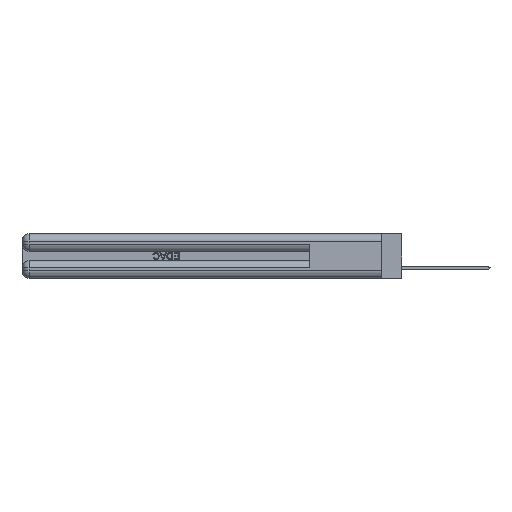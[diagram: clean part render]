
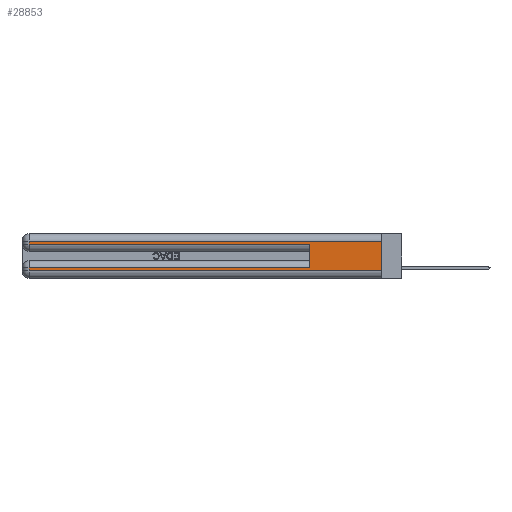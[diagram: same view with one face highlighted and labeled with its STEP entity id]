
A CAD part, left-side view. The second image highlights one B-rep face of the part: STEP entity #28853.
In plain terms, the highlighted planar face has unit normal (-1, 0, 0).
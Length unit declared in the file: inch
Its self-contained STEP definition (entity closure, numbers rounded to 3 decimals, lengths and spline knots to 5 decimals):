
#26 = EDGE_CURVE ( 'NONE', #20165, #24539, #9355, .T. ) ;
#175 = LINE ( 'NONE', #1362, #8796 ) ;
#1362 = CARTESIAN_POINT ( 'NONE',  ( 0., 0., 0.06 ) ) ;
#1652 = CARTESIAN_POINT ( 'NONE',  ( 0., 0.6, 0.145 ) ) ;
#2796 = VECTOR ( 'NONE', #25248, 39.37008 ) ;
#2855 = LINE ( 'NONE', #46911, #2796 ) ;
#3890 = CARTESIAN_POINT ( 'NONE',  ( 0., 2.94, 0.085 ) ) ;
#4137 = PLANE ( 'NONE',  #33162 ) ;
#4166 = CARTESIAN_POINT ( 'NONE',  ( 0., 0., 0.31 ) ) ;
#4442 = EDGE_CURVE ( 'NONE', #18019, #33013, #18798, .T. ) ;
#5843 = VERTEX_POINT ( 'NONE', #46590 ) ;
#6129 = ORIENTED_EDGE ( 'NONE', *, *, #8748, .T. ) ;
#6466 = ORIENTED_EDGE ( 'NONE', *, *, #26, .T. ) ;
#6897 = VECTOR ( 'NONE', #45679, 39.37008 ) ;
#8748 = EDGE_CURVE ( 'NONE', #40566, #5843, #175, .T. ) ;
#8796 = VECTOR ( 'NONE', #26908, 39.37008 ) ;
#9355 = LINE ( 'NONE', #15048, #45819 ) ;
#10079 = VECTOR ( 'NONE', #32707, 39.37008 ) ;
#11359 = EDGE_CURVE ( 'NONE', #24539, #33013, #2855, .T. ) ;
#11821 = CARTESIAN_POINT ( 'NONE',  ( 0., 0.6, 0.285 ) ) ;
#12032 = VERTEX_POINT ( 'NONE', #4166 ) ;
#14096 = EDGE_CURVE ( 'NONE', #45176, #40566, #24363, .T. ) ;
#15048 = CARTESIAN_POINT ( 'NONE',  ( 0., 2.94, 0.37 ) ) ;
#16114 = CARTESIAN_POINT ( 'NONE',  ( 0., 2.94, 0.31 ) ) ;
#16391 = CARTESIAN_POINT ( 'NONE',  ( 0., 2.94, 0.285 ) ) ;
#16403 = CARTESIAN_POINT ( 'NONE',  ( 0., 0., 0.31 ) ) ;
#17459 = LINE ( 'NONE', #28506, #28303 ) ;
#18019 = VERTEX_POINT ( 'NONE', #44288 ) ;
#18798 = LINE ( 'NONE', #1652, #34132 ) ;
#20165 = VERTEX_POINT ( 'NONE', #16114 ) ;
#21291 = ORIENTED_EDGE ( 'NONE', *, *, #32254, .F. ) ;
#22382 = CARTESIAN_POINT ( 'NONE',  ( 0., 0., 0.085 ) ) ;
#22405 = CARTESIAN_POINT ( 'NONE',  ( 0., 2.94, 0.37 ) ) ;
#22888 = DIRECTION ( 'NONE',  ( 0., 0., -1. ) ) ;
#23059 = CARTESIAN_POINT ( 'NONE',  ( 0., 2.94, 0.06 ) ) ;
#23196 = VECTOR ( 'NONE', #22888, 39.37008 ) ;
#24363 = LINE ( 'NONE', #22405, #23196 ) ;
#24539 = VERTEX_POINT ( 'NONE', #16391 ) ;
#24967 = DIRECTION ( 'NONE',  ( 0., 0., -1. ) ) ;
#25248 = DIRECTION ( 'NONE',  ( 0., -1., 0. ) ) ;
#26908 = DIRECTION ( 'NONE',  ( 0., -1., 0. ) ) ;
#27142 = EDGE_LOOP ( 'NONE', ( #21291, #37948, #6466, #43757, #36891, #32863, #29038, #6129 ) ) ;
#27457 = LINE ( 'NONE', #16403, #6897 ) ;
#28303 = VECTOR ( 'NONE', #24967, 39.37008 ) ;
#28506 = CARTESIAN_POINT ( 'NONE',  ( 0., 0., 0.37 ) ) ;
#28853 = ADVANCED_FACE ( 'NONE', ( #35822 ), #4137, .F. ) ;
#29038 = ORIENTED_EDGE ( 'NONE', *, *, #14096, .T. ) ;
#32254 = EDGE_CURVE ( 'NONE', #12032, #5843, #17459, .T. ) ;
#32707 = DIRECTION ( 'NONE',  ( 0., 1., 0. ) ) ;
#32863 = ORIENTED_EDGE ( 'NONE', *, *, #44579, .T. ) ;
#33013 = VERTEX_POINT ( 'NONE', #11821 ) ;
#33162 = AXIS2_PLACEMENT_3D ( 'NONE', #36755, #43799, #36131 ) ;
#33592 = DIRECTION ( 'NONE',  ( 0., 0., -1. ) ) ;
#34132 = VECTOR ( 'NONE', #35074, 39.37008 ) ;
#35074 = DIRECTION ( 'NONE',  ( 0., 0., 1. ) ) ;
#35822 = FACE_OUTER_BOUND ( 'NONE', #27142, .T. ) ;
#36131 = DIRECTION ( 'NONE',  ( 0., 0., -1. ) ) ;
#36755 = CARTESIAN_POINT ( 'NONE',  ( 0., 0., 0.37 ) ) ;
#36891 = ORIENTED_EDGE ( 'NONE', *, *, #4442, .F. ) ;
#37948 = ORIENTED_EDGE ( 'NONE', *, *, #43307, .T. ) ;
#40566 = VERTEX_POINT ( 'NONE', #23059 ) ;
#43307 = EDGE_CURVE ( 'NONE', #12032, #20165, #27457, .T. ) ;
#43696 = LINE ( 'NONE', #22382, #10079 ) ;
#43757 = ORIENTED_EDGE ( 'NONE', *, *, #11359, .T. ) ;
#43799 = DIRECTION ( 'NONE',  ( 1., 0., 0. ) ) ;
#44288 = CARTESIAN_POINT ( 'NONE',  ( 0., 0.6, 0.085 ) ) ;
#44579 = EDGE_CURVE ( 'NONE', #18019, #45176, #43696, .T. ) ;
#45176 = VERTEX_POINT ( 'NONE', #3890 ) ;
#45679 = DIRECTION ( 'NONE',  ( 0., 1., 0. ) ) ;
#45819 = VECTOR ( 'NONE', #33592, 39.37008 ) ;
#46590 = CARTESIAN_POINT ( 'NONE',  ( 0., 0., 0.06 ) ) ;
#46911 = CARTESIAN_POINT ( 'NONE',  ( 0., 0., 0.285 ) ) ;
